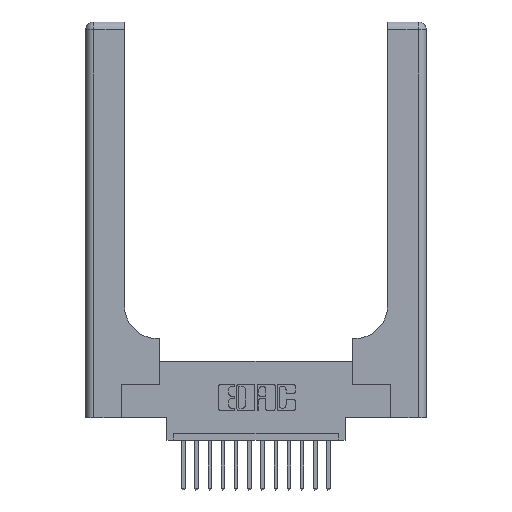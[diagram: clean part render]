
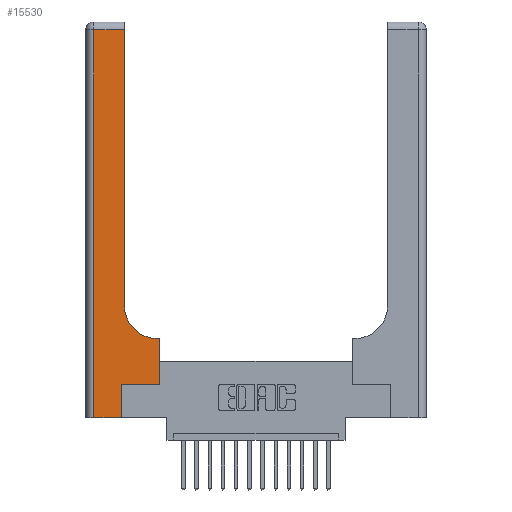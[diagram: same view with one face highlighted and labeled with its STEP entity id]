
A CAD part, top view. The second image highlights one B-rep face of the part: STEP entity #15530.
In plain terms, the highlighted planar face has unit normal (0, 0, 1).
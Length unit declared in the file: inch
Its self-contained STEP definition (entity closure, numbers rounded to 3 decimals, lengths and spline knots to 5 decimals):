
#328 = VECTOR ( 'NONE', #3049, 39.37008 ) ;
#380 = ORIENTED_EDGE ( 'NONE', *, *, #17245, .T. ) ;
#717 = PLANE ( 'NONE',  #16285 ) ;
#945 = CARTESIAN_POINT ( 'NONE',  ( 0.5415, 0.6, 0.37 ) ) ;
#981 = CARTESIAN_POINT ( 'NONE',  ( 0., 0., 0.37 ) ) ;
#1006 = CARTESIAN_POINT ( 'NONE',  ( 0.269, 0., 0.37 ) ) ;
#1489 = EDGE_CURVE ( 'NONE', #5050, #17623, #1836, .T. ) ;
#1836 = LINE ( 'NONE', #6055, #16513 ) ;
#1880 = CARTESIAN_POINT ( 'NONE',  ( 0., 2.94, 0.37 ) ) ;
#2007 = DIRECTION ( 'NONE',  ( 1., 0., 0. ) ) ;
#2084 = CIRCLE ( 'NONE', #6575, 0.25 ) ;
#2743 = ORIENTED_EDGE ( 'NONE', *, *, #16370, .T. ) ;
#2758 = VERTEX_POINT ( 'NONE', #12229 ) ;
#3049 = DIRECTION ( 'NONE',  ( -1., 0., 0. ) ) ;
#3301 = LINE ( 'NONE', #5806, #10664 ) ;
#3895 = LINE ( 'NONE', #1880, #328 ) ;
#5050 = VERTEX_POINT ( 'NONE', #13099 ) ;
#5278 = VERTEX_POINT ( 'NONE', #17916 ) ;
#5404 = EDGE_CURVE ( 'NONE', #5278, #12098, #7746, .T. ) ;
#5513 = EDGE_CURVE ( 'NONE', #7508, #11720, #5923, .T. ) ;
#5532 = VECTOR ( 'NONE', #11667, 39.37008 ) ;
#5660 = ORIENTED_EDGE ( 'NONE', *, *, #5513, .T. ) ;
#5806 = CARTESIAN_POINT ( 'NONE',  ( 0.06, 3., 0.37 ) ) ;
#5923 = LINE ( 'NONE', #13459, #9955 ) ;
#6055 = CARTESIAN_POINT ( 'NONE',  ( 0.2915, 3., 0.37 ) ) ;
#6127 = VECTOR ( 'NONE', #18092, 39.37008 ) ;
#6575 = AXIS2_PLACEMENT_3D ( 'NONE', #15704, #17080, #11421 ) ;
#6647 = CARTESIAN_POINT ( 'NONE',  ( 0.06, 0., 0.37 ) ) ;
#6770 = EDGE_CURVE ( 'NONE', #12098, #5050, #2084, .T. ) ;
#7023 = EDGE_CURVE ( 'NONE', #11720, #5278, #12652, .T. ) ;
#7038 = DIRECTION ( 'NONE',  ( -1., 0., 0. ) ) ;
#7290 = CARTESIAN_POINT ( 'NONE',  ( 0.2915, 0.6, 0.37 ) ) ;
#7323 = CARTESIAN_POINT ( 'NONE',  ( 0.5585, 0.25, 0.37 ) ) ;
#7486 = LINE ( 'NONE', #1006, #6127 ) ;
#7508 = VERTEX_POINT ( 'NONE', #17489 ) ;
#7518 = ORIENTED_EDGE ( 'NONE', *, *, #1489, .T. ) ;
#7695 = CARTESIAN_POINT ( 'NONE',  ( 0.06, 2.94, 0.37 ) ) ;
#7717 = CARTESIAN_POINT ( 'NONE',  ( 0.2915, 2.94, 0.37 ) ) ;
#7746 = LINE ( 'NONE', #7290, #12386 ) ;
#7847 = DIRECTION ( 'NONE',  ( 0., 0., -1. ) ) ;
#7856 = ORIENTED_EDGE ( 'NONE', *, *, #9798, .T. ) ;
#8521 = ORIENTED_EDGE ( 'NONE', *, *, #7023, .T. ) ;
#9490 = EDGE_CURVE ( 'NONE', #2758, #7508, #7486, .T. ) ;
#9798 = EDGE_CURVE ( 'NONE', #17623, #16551, #3895, .T. ) ;
#9955 = VECTOR ( 'NONE', #2007, 39.37008 ) ;
#10467 = ORIENTED_EDGE ( 'NONE', *, *, #9490, .T. ) ;
#10664 = VECTOR ( 'NONE', #15740, 39.37008 ) ;
#11421 = DIRECTION ( 'NONE',  ( 1., 0., 0. ) ) ;
#11667 = DIRECTION ( 'NONE',  ( 0., 1., 0. ) ) ;
#11720 = VERTEX_POINT ( 'NONE', #7323 ) ;
#12098 = VERTEX_POINT ( 'NONE', #945 ) ;
#12229 = CARTESIAN_POINT ( 'NONE',  ( 0.269, 0., 0.37 ) ) ;
#12386 = VECTOR ( 'NONE', #7038, 39.37008 ) ;
#12403 = LINE ( 'NONE', #981, #17286 ) ;
#12652 = LINE ( 'NONE', #14678, #5532 ) ;
#13099 = CARTESIAN_POINT ( 'NONE',  ( 0.2915, 0.85, 0.37 ) ) ;
#13395 = DIRECTION ( 'NONE',  ( 0., 1., 0. ) ) ;
#13459 = CARTESIAN_POINT ( 'NONE',  ( 0.269, 0.25, 0.37 ) ) ;
#13737 = DIRECTION ( 'NONE',  ( 1., 0., 0. ) ) ;
#14678 = CARTESIAN_POINT ( 'NONE',  ( 0.5585, 0.25, 0.37 ) ) ;
#14837 = CARTESIAN_POINT ( 'NONE',  ( 0., 3., 0.37 ) ) ;
#14844 = ORIENTED_EDGE ( 'NONE', *, *, #5404, .T. ) ;
#15530 = ADVANCED_FACE ( 'NONE', ( #16695 ), #717, .F. ) ;
#15594 = EDGE_LOOP ( 'NONE', ( #7518, #7856, #2743, #380, #10467, #5660, #8521, #14844, #17499 ) ) ;
#15704 = CARTESIAN_POINT ( 'NONE',  ( 0.5415, 0.85, 0.37 ) ) ;
#15740 = DIRECTION ( 'NONE',  ( 0., -1., 0. ) ) ;
#16285 = AXIS2_PLACEMENT_3D ( 'NONE', #14837, #7847, #17866 ) ;
#16370 = EDGE_CURVE ( 'NONE', #16551, #17236, #3301, .T. ) ;
#16513 = VECTOR ( 'NONE', #13395, 39.37008 ) ;
#16551 = VERTEX_POINT ( 'NONE', #7695 ) ;
#16695 = FACE_OUTER_BOUND ( 'NONE', #15594, .T. ) ;
#17080 = DIRECTION ( 'NONE',  ( 0., 0., -1. ) ) ;
#17236 = VERTEX_POINT ( 'NONE', #6647 ) ;
#17245 = EDGE_CURVE ( 'NONE', #17236, #2758, #12403, .T. ) ;
#17286 = VECTOR ( 'NONE', #13737, 39.37008 ) ;
#17489 = CARTESIAN_POINT ( 'NONE',  ( 0.269, 0.25, 0.37 ) ) ;
#17499 = ORIENTED_EDGE ( 'NONE', *, *, #6770, .T. ) ;
#17623 = VERTEX_POINT ( 'NONE', #7717 ) ;
#17866 = DIRECTION ( 'NONE',  ( -1., 0., 0. ) ) ;
#17916 = CARTESIAN_POINT ( 'NONE',  ( 0.5585, 0.6, 0.37 ) ) ;
#18092 = DIRECTION ( 'NONE',  ( 0., 1., 0. ) ) ;
